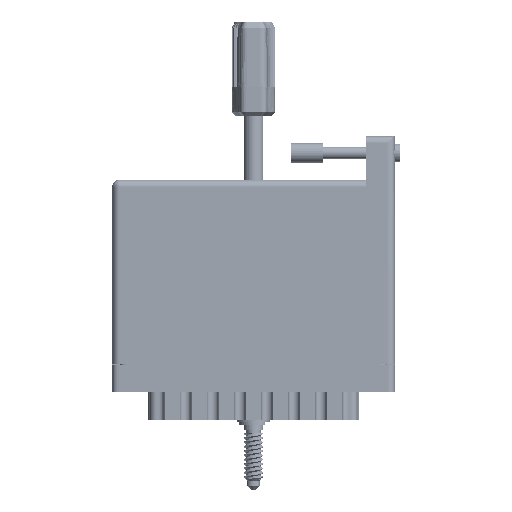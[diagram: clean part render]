
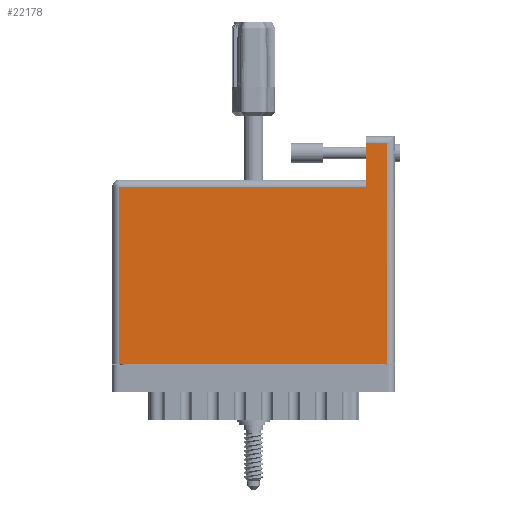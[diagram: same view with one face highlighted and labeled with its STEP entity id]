
A CAD part, front view. The second image highlights one B-rep face of the part: STEP entity #22178.
In plain terms, the highlighted face is planar.
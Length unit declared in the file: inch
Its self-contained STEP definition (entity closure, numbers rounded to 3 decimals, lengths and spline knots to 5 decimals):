
#992 = FACE_OUTER_BOUND ( 'NONE', #57799, .T. ) ;
#4432 = DIRECTION ( 'NONE',  ( -1., 0., 0. ) ) ;
#7261 = CARTESIAN_POINT ( 'NONE',  ( 2.648, 2.125, 0. ) ) ;
#8085 = CARTESIAN_POINT ( 'NONE',  ( 2.438, 2.195, 0. ) ) ;
#8247 = VECTOR ( 'NONE', #48442, 39.37008 ) ;
#8270 = VECTOR ( 'NONE', #83067, 39.37008 ) ;
#14578 = EDGE_CURVE ( 'NONE', #27282, #75794, #22282, .T. ) ;
#14703 = CARTESIAN_POINT ( 'NONE',  ( 2.438, 2.125, 0. ) ) ;
#16154 = LINE ( 'NONE', #39873, #52731 ) ;
#20129 = CARTESIAN_POINT ( 'NONE',  ( 0., 1.775, 0. ) ) ;
#21654 = CARTESIAN_POINT ( 'NONE',  ( 2.648, 2.195, 0. ) ) ;
#21668 = ORIENTED_EDGE ( 'NONE', *, *, #14578, .T. ) ;
#22178 = ADVANCED_FACE ( 'NONE', ( #992 ), #54996, .F. ) ;
#22282 = LINE ( 'NONE', #46705, #8270 ) ;
#22312 = EDGE_CURVE ( 'NONE', #75794, #59265, #68957, .T. ) ;
#23399 = EDGE_CURVE ( 'NONE', #79871, #84910, #53542, .T. ) ;
#25513 = VERTEX_POINT ( 'NONE', #63654 ) ;
#25522 = LINE ( 'NONE', #21654, #8247 ) ;
#27282 = VERTEX_POINT ( 'NONE', #82178 ) ;
#29223 = EDGE_CURVE ( 'NONE', #25513, #79871, #25522, .T. ) ;
#29522 = LINE ( 'NONE', #8085, #84430 ) ;
#31313 = CARTESIAN_POINT ( 'NONE',  ( 0., 2.125, 0. ) ) ;
#38452 = ORIENTED_EDGE ( 'NONE', *, *, #22312, .T. ) ;
#39873 = CARTESIAN_POINT ( 'NONE',  ( 0., 0., 0. ) ) ;
#41110 = DIRECTION ( 'NONE',  ( -1., 0., 0. ) ) ;
#46705 = CARTESIAN_POINT ( 'NONE',  ( 0., 1.705, 0. ) ) ;
#48442 = DIRECTION ( 'NONE',  ( 0., 1., 0. ) ) ;
#50639 = VECTOR ( 'NONE', #88401, 39.37008 ) ;
#52731 = VECTOR ( 'NONE', #81745, 39.37008 ) ;
#53280 = EDGE_CURVE ( 'NONE', #59265, #25513, #16154, .T. ) ;
#53542 = LINE ( 'NONE', #31313, #66546 ) ;
#54996 = PLANE ( 'NONE',  #84831 ) ;
#55355 = DIRECTION ( 'NONE',  ( 0., -1., 0. ) ) ;
#57799 = EDGE_LOOP ( 'NONE', ( #21668, #38452, #67493, #84295, #79416, #82744 ) ) ;
#59265 = VERTEX_POINT ( 'NONE', #75027 ) ;
#63654 = CARTESIAN_POINT ( 'NONE',  ( 2.648, 0., 0. ) ) ;
#66546 = VECTOR ( 'NONE', #4432, 39.37008 ) ;
#67493 = ORIENTED_EDGE ( 'NONE', *, *, #53280, .T. ) ;
#68887 = DIRECTION ( 'NONE',  ( 0., 0., -1. ) ) ;
#68957 = LINE ( 'NONE', #88106, #50639 ) ;
#75027 = CARTESIAN_POINT ( 'NONE',  ( 0.07, 0., 0. ) ) ;
#75794 = VERTEX_POINT ( 'NONE', #89241 ) ;
#78560 = EDGE_CURVE ( 'NONE', #84910, #27282, #29522, .T. ) ;
#79416 = ORIENTED_EDGE ( 'NONE', *, *, #23399, .T. ) ;
#79871 = VERTEX_POINT ( 'NONE', #7261 ) ;
#81745 = DIRECTION ( 'NONE',  ( 1., 0., 0. ) ) ;
#82178 = CARTESIAN_POINT ( 'NONE',  ( 2.438, 1.705, 0. ) ) ;
#82744 = ORIENTED_EDGE ( 'NONE', *, *, #78560, .T. ) ;
#83067 = DIRECTION ( 'NONE',  ( -1., 0., 0. ) ) ;
#84295 = ORIENTED_EDGE ( 'NONE', *, *, #29223, .T. ) ;
#84430 = VECTOR ( 'NONE', #55355, 39.37008 ) ;
#84831 = AXIS2_PLACEMENT_3D ( 'NONE', #20129, #68887, #41110 ) ;
#84910 = VERTEX_POINT ( 'NONE', #14703 ) ;
#88106 = CARTESIAN_POINT ( 'NONE',  ( 0.07, 0., 0. ) ) ;
#88401 = DIRECTION ( 'NONE',  ( 0., -1., 0. ) ) ;
#89241 = CARTESIAN_POINT ( 'NONE',  ( 0.07, 1.705, 0. ) ) ;
